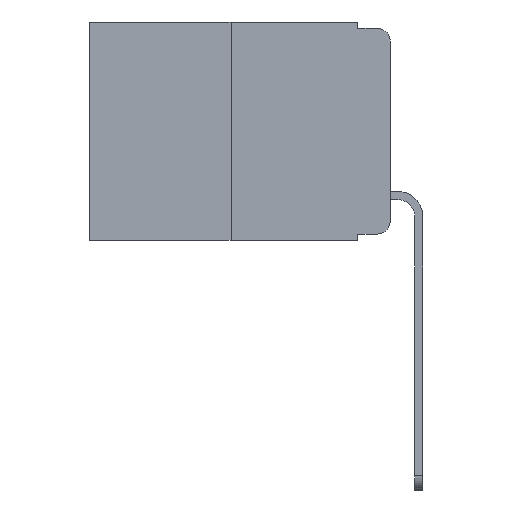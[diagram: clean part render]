
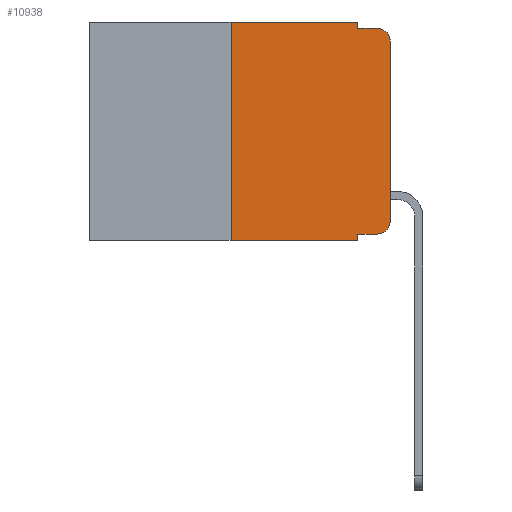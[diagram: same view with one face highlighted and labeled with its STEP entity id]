
A CAD part, left-side view. The second image highlights one B-rep face of the part: STEP entity #10938.
In plain terms, the highlighted planar face has unit normal (-1, 0, 0).
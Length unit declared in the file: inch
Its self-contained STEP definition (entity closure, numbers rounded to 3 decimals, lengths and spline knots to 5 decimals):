
#30 = VERTEX_POINT ( 'NONE', #1764 ) ;
#412 = CARTESIAN_POINT ( 'NONE',  ( 0., 0.051, -0.01 ) ) ;
#433 = CARTESIAN_POINT ( 'NONE',  ( 0., 0., -0.03 ) ) ;
#982 = EDGE_CURVE ( 'NONE', #3763, #10269, #1997, .T. ) ;
#1140 = VERTEX_POINT ( 'NONE', #12762 ) ;
#1224 = DIRECTION ( 'NONE',  ( 0., -1., 0. ) ) ;
#1246 = ORIENTED_EDGE ( 'NONE', *, *, #12862, .T. ) ;
#1504 = CIRCLE ( 'NONE', #11243, 0.02 ) ;
#1627 = LINE ( 'NONE', #412, #6176 ) ;
#1764 = CARTESIAN_POINT ( 'NONE',  ( 0., 0.02, -0.01 ) ) ;
#1799 = VERTEX_POINT ( 'NONE', #6744 ) ;
#1977 = ORIENTED_EDGE ( 'NONE', *, *, #3420, .F. ) ;
#1997 = LINE ( 'NONE', #6495, #4214 ) ;
#2080 = LINE ( 'NONE', #5491, #5841 ) ;
#2107 = AXIS2_PLACEMENT_3D ( 'NONE', #2241, #11297, #12156 ) ;
#2241 = CARTESIAN_POINT ( 'NONE',  ( 0., 0.02, -0.313 ) ) ;
#2458 = ORIENTED_EDGE ( 'NONE', *, *, #5258, .F. ) ;
#2552 = CARTESIAN_POINT ( 'NONE',  ( 0., 0.051, 0. ) ) ;
#2669 = ORIENTED_EDGE ( 'NONE', *, *, #5703, .T. ) ;
#2873 = CARTESIAN_POINT ( 'NONE',  ( 0., 0.051, -0.333 ) ) ;
#2885 = CIRCLE ( 'NONE', #2107, 0.02 ) ;
#3420 = EDGE_CURVE ( 'NONE', #1140, #1799, #4171, .T. ) ;
#3555 = DIRECTION ( 'NONE',  ( 0., 0., 1. ) ) ;
#3685 = LINE ( 'NONE', #10266, #4317 ) ;
#3700 = CARTESIAN_POINT ( 'NONE',  ( 0., 0.473, 0. ) ) ;
#3763 = VERTEX_POINT ( 'NONE', #6092 ) ;
#4120 = DIRECTION ( 'NONE',  ( -1., 0., 0. ) ) ;
#4150 = VECTOR ( 'NONE', #1224, 39.37008 ) ;
#4171 = LINE ( 'NONE', #2552, #12536 ) ;
#4214 = VECTOR ( 'NONE', #3555, 39.37008 ) ;
#4252 = DIRECTION ( 'NONE',  ( 0., 0., 1. ) ) ;
#4317 = VECTOR ( 'NONE', #4252, 39.37008 ) ;
#4366 = DIRECTION ( 'NONE',  ( 0., -1., 0. ) ) ;
#4381 = VECTOR ( 'NONE', #4366, 39.37008 ) ;
#4852 = CARTESIAN_POINT ( 'NONE',  ( 0., 0., -0.313 ) ) ;
#5202 = AXIS2_PLACEMENT_3D ( 'NONE', #3700, #6640, #11665 ) ;
#5258 = EDGE_CURVE ( 'NONE', #1799, #30, #1627, .T. ) ;
#5270 = LINE ( 'NONE', #9594, #7637 ) ;
#5289 = ORIENTED_EDGE ( 'NONE', *, *, #982, .F. ) ;
#5356 = VERTEX_POINT ( 'NONE', #11613 ) ;
#5459 = EDGE_CURVE ( 'NONE', #10269, #1140, #2080, .T. ) ;
#5491 = CARTESIAN_POINT ( 'NONE',  ( 0., 0.473, 0. ) ) ;
#5703 = EDGE_CURVE ( 'NONE', #11589, #12400, #3685, .T. ) ;
#5841 = VECTOR ( 'NONE', #12008, 39.37008 ) ;
#5861 = EDGE_CURVE ( 'NONE', #3763, #5356, #12520, .T. ) ;
#5936 = ORIENTED_EDGE ( 'NONE', *, *, #10691, .T. ) ;
#6092 = CARTESIAN_POINT ( 'NONE',  ( 0., 0.25, -0.343 ) ) ;
#6176 = VECTOR ( 'NONE', #10455, 39.37008 ) ;
#6249 = FACE_OUTER_BOUND ( 'NONE', #6457, .T. ) ;
#6290 = VERTEX_POINT ( 'NONE', #2873 ) ;
#6457 = EDGE_LOOP ( 'NONE', ( #2669, #8289, #2458, #1977, #7237, #5289, #8435, #8054, #5936, #1246 ) ) ;
#6495 = CARTESIAN_POINT ( 'NONE',  ( 0., 0.25, 0. ) ) ;
#6640 = DIRECTION ( 'NONE',  ( 1., 0., 0. ) ) ;
#6744 = CARTESIAN_POINT ( 'NONE',  ( 0., 0.051, -0.01 ) ) ;
#7237 = ORIENTED_EDGE ( 'NONE', *, *, #5459, .F. ) ;
#7422 = CARTESIAN_POINT ( 'NONE',  ( 0., 0.051, -0.333 ) ) ;
#7637 = VECTOR ( 'NONE', #8660, 39.37008 ) ;
#8054 = ORIENTED_EDGE ( 'NONE', *, *, #12554, .F. ) ;
#8071 = VERTEX_POINT ( 'NONE', #8672 ) ;
#8289 = ORIENTED_EDGE ( 'NONE', *, *, #8540, .T. ) ;
#8435 = ORIENTED_EDGE ( 'NONE', *, *, #5861, .T. ) ;
#8540 = EDGE_CURVE ( 'NONE', #12400, #30, #1504, .T. ) ;
#8660 = DIRECTION ( 'NONE',  ( 0., 0., -1. ) ) ;
#8672 = CARTESIAN_POINT ( 'NONE',  ( 0., 0.02, -0.333 ) ) ;
#9590 = DIRECTION ( 'NONE',  ( 0., 0., -1. ) ) ;
#9594 = CARTESIAN_POINT ( 'NONE',  ( 0., 0.051, 0. ) ) ;
#10266 = CARTESIAN_POINT ( 'NONE',  ( 0., 0., 0. ) ) ;
#10269 = VERTEX_POINT ( 'NONE', #13076 ) ;
#10455 = DIRECTION ( 'NONE',  ( 0., -1., 0. ) ) ;
#10691 = EDGE_CURVE ( 'NONE', #6290, #8071, #11777, .T. ) ;
#10938 = ADVANCED_FACE ( 'NONE', ( #6249 ), #12867, .F. ) ;
#11136 = DIRECTION ( 'NONE',  ( 0., 0., -1. ) ) ;
#11243 = AXIS2_PLACEMENT_3D ( 'NONE', #12372, #4120, #11136 ) ;
#11297 = DIRECTION ( 'NONE',  ( -1., 0., 0. ) ) ;
#11419 = CARTESIAN_POINT ( 'NONE',  ( 0., 0.473, -0.343 ) ) ;
#11589 = VERTEX_POINT ( 'NONE', #4852 ) ;
#11613 = CARTESIAN_POINT ( 'NONE',  ( 0., 0.051, -0.343 ) ) ;
#11665 = DIRECTION ( 'NONE',  ( 0., 0., -1. ) ) ;
#11777 = LINE ( 'NONE', #7422, #4381 ) ;
#12008 = DIRECTION ( 'NONE',  ( 0., -1., 0. ) ) ;
#12156 = DIRECTION ( 'NONE',  ( 0., 0., -1. ) ) ;
#12372 = CARTESIAN_POINT ( 'NONE',  ( 0., 0.02, -0.03 ) ) ;
#12400 = VERTEX_POINT ( 'NONE', #433 ) ;
#12520 = LINE ( 'NONE', #11419, #4150 ) ;
#12536 = VECTOR ( 'NONE', #9590, 39.37008 ) ;
#12554 = EDGE_CURVE ( 'NONE', #6290, #5356, #5270, .T. ) ;
#12762 = CARTESIAN_POINT ( 'NONE',  ( 0., 0.051, 0. ) ) ;
#12862 = EDGE_CURVE ( 'NONE', #8071, #11589, #2885, .T. ) ;
#12867 = PLANE ( 'NONE',  #5202 ) ;
#13076 = CARTESIAN_POINT ( 'NONE',  ( 0., 0.25, 0. ) ) ;
